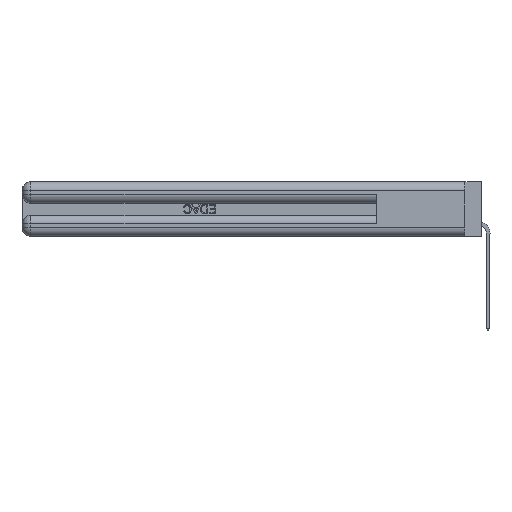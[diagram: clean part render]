
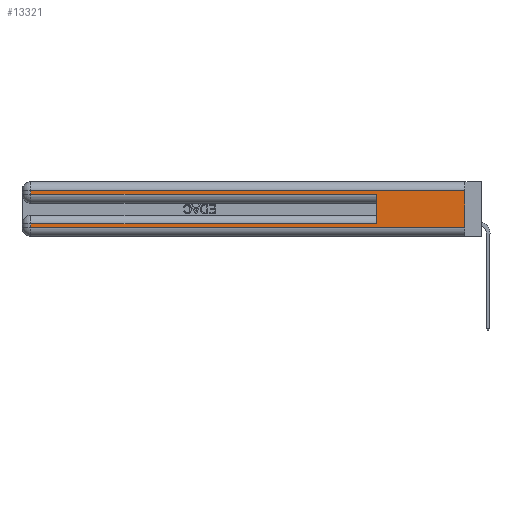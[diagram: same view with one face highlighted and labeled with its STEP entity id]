
A CAD part, left-side view. The second image highlights one B-rep face of the part: STEP entity #13321.
In plain terms, the highlighted planar face has unit normal (-1, 0, 0).
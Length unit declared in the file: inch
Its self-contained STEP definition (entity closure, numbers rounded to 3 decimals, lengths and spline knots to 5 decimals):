
#659 = EDGE_CURVE ( 'NONE', #5405, #15639, #15950, .T. ) ;
#2595 = CARTESIAN_POINT ( 'NONE',  ( 0., 0.6, 0.145 ) ) ;
#3136 = CARTESIAN_POINT ( 'NONE',  ( 0., 0.6, 0.285 ) ) ;
#3404 = CARTESIAN_POINT ( 'NONE',  ( 0., 0., 0.06 ) ) ;
#4302 = VERTEX_POINT ( 'NONE', #4471 ) ;
#4471 = CARTESIAN_POINT ( 'NONE',  ( 0., 2.94, 0.31 ) ) ;
#4638 = VECTOR ( 'NONE', #5197, 39.37008 ) ;
#4669 = CARTESIAN_POINT ( 'NONE',  ( 0., 0.6, 0.085 ) ) ;
#4826 = LINE ( 'NONE', #14334, #16179 ) ;
#4937 = DIRECTION ( 'NONE',  ( 0., 0., -1. ) ) ;
#5197 = DIRECTION ( 'NONE',  ( 0., -1., 0. ) ) ;
#5405 = VERTEX_POINT ( 'NONE', #4669 ) ;
#5971 = VERTEX_POINT ( 'NONE', #3404 ) ;
#6175 = CARTESIAN_POINT ( 'NONE',  ( 0., 0., 0.31 ) ) ;
#8053 = LINE ( 'NONE', #16105, #17876 ) ;
#8475 = VERTEX_POINT ( 'NONE', #21904 ) ;
#8743 = LINE ( 'NONE', #16831, #12876 ) ;
#8931 = AXIS2_PLACEMENT_3D ( 'NONE', #30137, #22395, #32857 ) ;
#9005 = LINE ( 'NONE', #20082, #27435 ) ;
#9785 = EDGE_CURVE ( 'NONE', #19812, #4302, #8053, .T. ) ;
#9941 = EDGE_CURVE ( 'NONE', #5405, #13483, #31042, .T. ) ;
#10690 = ORIENTED_EDGE ( 'NONE', *, *, #9941, .F. ) ;
#11216 = DIRECTION ( 'NONE',  ( 0., 1., 0. ) ) ;
#11780 = PLANE ( 'NONE',  #8931 ) ;
#12876 = VECTOR ( 'NONE', #14482, 39.37008 ) ;
#13143 = LINE ( 'NONE', #28160, #29115 ) ;
#13321 = ADVANCED_FACE ( 'NONE', ( #30051 ), #11780, .F. ) ;
#13483 = VERTEX_POINT ( 'NONE', #3136 ) ;
#14334 = CARTESIAN_POINT ( 'NONE',  ( 0., 2.94, 0.37 ) ) ;
#14482 = DIRECTION ( 'NONE',  ( 0., -1., 0. ) ) ;
#14753 = EDGE_CURVE ( 'NONE', #4302, #8475, #9005, .T. ) ;
#15624 = CARTESIAN_POINT ( 'NONE',  ( 0., 2.94, 0.085 ) ) ;
#15639 = VERTEX_POINT ( 'NONE', #15624 ) ;
#15950 = LINE ( 'NONE', #21650, #32389 ) ;
#16105 = CARTESIAN_POINT ( 'NONE',  ( 0., 0., 0.31 ) ) ;
#16149 = ORIENTED_EDGE ( 'NONE', *, *, #16621, .T. ) ;
#16179 = VECTOR ( 'NONE', #16794, 39.37008 ) ;
#16621 = EDGE_CURVE ( 'NONE', #15639, #25352, #4826, .T. ) ;
#16794 = DIRECTION ( 'NONE',  ( 0., 0., -1. ) ) ;
#16831 = CARTESIAN_POINT ( 'NONE',  ( 0., 0., 0.06 ) ) ;
#17412 = ORIENTED_EDGE ( 'NONE', *, *, #33377, .F. ) ;
#17876 = VECTOR ( 'NONE', #11216, 39.37008 ) ;
#18429 = ORIENTED_EDGE ( 'NONE', *, *, #14753, .T. ) ;
#18620 = CARTESIAN_POINT ( 'NONE',  ( 0., 2.94, 0.06 ) ) ;
#18839 = LINE ( 'NONE', #31079, #4638 ) ;
#19134 = ORIENTED_EDGE ( 'NONE', *, *, #659, .T. ) ;
#19241 = DIRECTION ( 'NONE',  ( 0., 1., 0. ) ) ;
#19812 = VERTEX_POINT ( 'NONE', #6175 ) ;
#20082 = CARTESIAN_POINT ( 'NONE',  ( 0., 2.94, 0.37 ) ) ;
#21650 = CARTESIAN_POINT ( 'NONE',  ( 0., 0., 0.085 ) ) ;
#21904 = CARTESIAN_POINT ( 'NONE',  ( 0., 2.94, 0.285 ) ) ;
#22395 = DIRECTION ( 'NONE',  ( 1., 0., 0. ) ) ;
#24522 = ORIENTED_EDGE ( 'NONE', *, *, #25496, .T. ) ;
#25178 = DIRECTION ( 'NONE',  ( 0., 0., -1. ) ) ;
#25306 = ORIENTED_EDGE ( 'NONE', *, *, #9785, .T. ) ;
#25352 = VERTEX_POINT ( 'NONE', #18620 ) ;
#25496 = EDGE_CURVE ( 'NONE', #25352, #5971, #8743, .T. ) ;
#25687 = VECTOR ( 'NONE', #26125, 39.37008 ) ;
#26125 = DIRECTION ( 'NONE',  ( 0., 0., 1. ) ) ;
#27435 = VECTOR ( 'NONE', #25178, 39.37008 ) ;
#27449 = EDGE_CURVE ( 'NONE', #8475, #13483, #18839, .T. ) ;
#28160 = CARTESIAN_POINT ( 'NONE',  ( 0., 0., 0.37 ) ) ;
#29115 = VECTOR ( 'NONE', #4937, 39.37008 ) ;
#29151 = ORIENTED_EDGE ( 'NONE', *, *, #27449, .T. ) ;
#29194 = EDGE_LOOP ( 'NONE', ( #17412, #25306, #18429, #29151, #10690, #19134, #16149, #24522 ) ) ;
#30051 = FACE_OUTER_BOUND ( 'NONE', #29194, .T. ) ;
#30137 = CARTESIAN_POINT ( 'NONE',  ( 0., 0., 0.37 ) ) ;
#31042 = LINE ( 'NONE', #2595, #25687 ) ;
#31079 = CARTESIAN_POINT ( 'NONE',  ( 0., 0., 0.285 ) ) ;
#32389 = VECTOR ( 'NONE', #19241, 39.37008 ) ;
#32857 = DIRECTION ( 'NONE',  ( 0., 0., -1. ) ) ;
#33377 = EDGE_CURVE ( 'NONE', #19812, #5971, #13143, .T. ) ;
